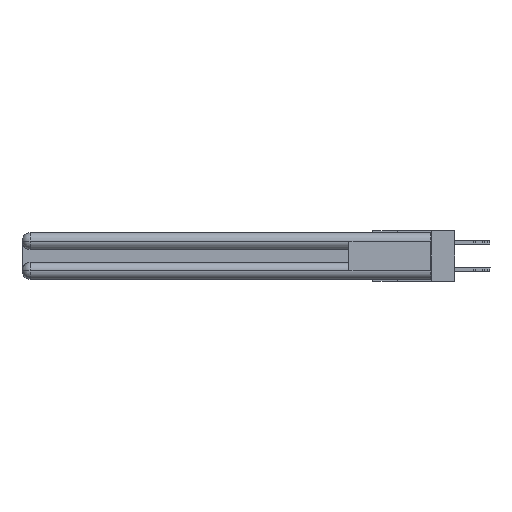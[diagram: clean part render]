
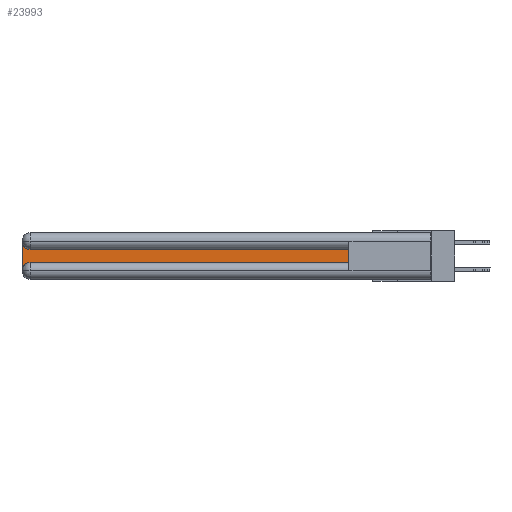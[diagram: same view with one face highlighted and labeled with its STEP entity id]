
A CAD part, left-side view. The second image highlights one B-rep face of the part: STEP entity #23993.
In plain terms, the highlighted planar face has unit normal (-1, 0, 0).
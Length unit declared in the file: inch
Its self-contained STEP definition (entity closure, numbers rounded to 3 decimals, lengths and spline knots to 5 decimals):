
#185 = LINE ( 'NONE', #12097, #26140 ) ;
#909 = EDGE_CURVE ( 'NONE', #23761, #29028, #34591, .T. ) ;
#964 = DIRECTION ( 'NONE',  ( 0., 0., -1. ) ) ;
#1115 = ORIENTED_EDGE ( 'NONE', *, *, #3926, .T. ) ;
#1918 = VERTEX_POINT ( 'NONE', #28681 ) ;
#2582 = VECTOR ( 'NONE', #30655, 39.37008 ) ;
#3029 = EDGE_CURVE ( 'NONE', #29028, #1918, #5123, .T. ) ;
#3926 = EDGE_CURVE ( 'NONE', #1918, #26396, #21408, .T. ) ;
#4201 = CARTESIAN_POINT ( 'NONE',  ( 0.075, 0.6, -0.2175 ) ) ;
#5123 = CIRCLE ( 'NONE', #13672, 0.06 ) ;
#5436 = VERTEX_POINT ( 'NONE', #21580 ) ;
#5463 = EDGE_CURVE ( 'NONE', #26396, #5436, #26371, .T. ) ;
#5526 = DIRECTION ( 'NONE',  ( 0., 0., -1. ) ) ;
#5818 = CARTESIAN_POINT ( 'NONE',  ( 0.075, 0.6, -0.1225 ) ) ;
#5845 = DIRECTION ( 'NONE',  ( 1., 0., 0. ) ) ;
#6088 = ORIENTED_EDGE ( 'NONE', *, *, #909, .T. ) ;
#6097 = AXIS2_PLACEMENT_3D ( 'NONE', #34429, #29509, #5526 ) ;
#11151 = DIRECTION ( 'NONE',  ( 0., 0., -1. ) ) ;
#11624 = DIRECTION ( 'NONE',  ( 1., 0., 0. ) ) ;
#12097 = CARTESIAN_POINT ( 'NONE',  ( 0.075, 0.6, -0.2175 ) ) ;
#13672 = AXIS2_PLACEMENT_3D ( 'NONE', #32983, #5845, #964 ) ;
#13975 = EDGE_CURVE ( 'NONE', #5436, #15189, #23548, .T. ) ;
#14014 = ORIENTED_EDGE ( 'NONE', *, *, #31389, .T. ) ;
#14231 = DIRECTION ( 'NONE',  ( 0., 1., 0. ) ) ;
#15189 = VERTEX_POINT ( 'NONE', #27634 ) ;
#17014 = DIRECTION ( 'NONE',  ( 0., 0., -1. ) ) ;
#17746 = ORIENTED_EDGE ( 'NONE', *, *, #5463, .T. ) ;
#19384 = EDGE_LOOP ( 'NONE', ( #6088, #25784, #1115, #17746, #25329, #14014 ) ) ;
#19563 = CARTESIAN_POINT ( 'NONE',  ( 0.075, 3., -0.2775 ) ) ;
#21408 = LINE ( 'NONE', #33398, #22233 ) ;
#21580 = CARTESIAN_POINT ( 'NONE',  ( 0.075, 2.94, -0.2175 ) ) ;
#22233 = VECTOR ( 'NONE', #11151, 39.37008 ) ;
#23548 = LINE ( 'NONE', #4201, #2582 ) ;
#23761 = VERTEX_POINT ( 'NONE', #29019 ) ;
#23993 = ADVANCED_FACE ( 'NONE', ( #33898 ), #33144, .F. ) ;
#25329 = ORIENTED_EDGE ( 'NONE', *, *, #13975, .T. ) ;
#25452 = CARTESIAN_POINT ( 'NONE',  ( 0.075, 2.94, -0.1225 ) ) ;
#25784 = ORIENTED_EDGE ( 'NONE', *, *, #3029, .T. ) ;
#26140 = VECTOR ( 'NONE', #29148, 39.37008 ) ;
#26371 = CIRCLE ( 'NONE', #6097, 0.06 ) ;
#26396 = VERTEX_POINT ( 'NONE', #19563 ) ;
#27634 = CARTESIAN_POINT ( 'NONE',  ( 0.075, 0.6, -0.2175 ) ) ;
#27635 = CARTESIAN_POINT ( 'NONE',  ( 0.075, 3., -0.1225 ) ) ;
#28681 = CARTESIAN_POINT ( 'NONE',  ( 0.075, 3., -0.0625 ) ) ;
#29019 = CARTESIAN_POINT ( 'NONE',  ( 0.075, 0.6, -0.1225 ) ) ;
#29028 = VERTEX_POINT ( 'NONE', #25452 ) ;
#29148 = DIRECTION ( 'NONE',  ( 0., 0., 1. ) ) ;
#29509 = DIRECTION ( 'NONE',  ( 1., 0., 0. ) ) ;
#30655 = DIRECTION ( 'NONE',  ( 0., -1., 0. ) ) ;
#31221 = VECTOR ( 'NONE', #14231, 39.37008 ) ;
#31389 = EDGE_CURVE ( 'NONE', #15189, #23761, #185, .T. ) ;
#32983 = CARTESIAN_POINT ( 'NONE',  ( 0.075, 2.94, -0.0625 ) ) ;
#33144 = PLANE ( 'NONE',  #33229 ) ;
#33229 = AXIS2_PLACEMENT_3D ( 'NONE', #27635, #11624, #17014 ) ;
#33398 = CARTESIAN_POINT ( 'NONE',  ( 0.075, 3., -0.2175 ) ) ;
#33898 = FACE_OUTER_BOUND ( 'NONE', #19384, .T. ) ;
#34429 = CARTESIAN_POINT ( 'NONE',  ( 0.075, 2.94, -0.2775 ) ) ;
#34591 = LINE ( 'NONE', #5818, #31221 ) ;
